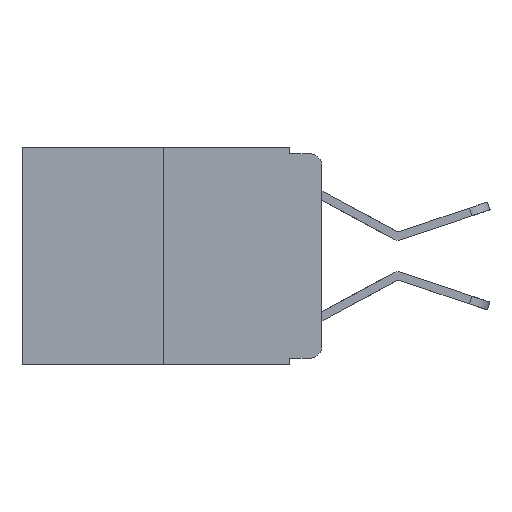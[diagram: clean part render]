
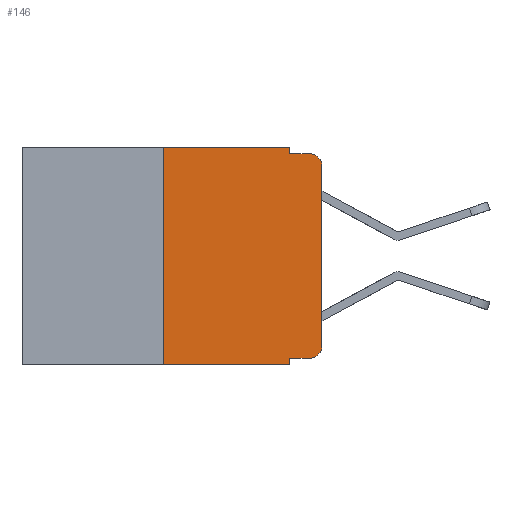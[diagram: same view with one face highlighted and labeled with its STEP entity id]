
A CAD part, left-side view. The second image highlights one B-rep face of the part: STEP entity #146.
In plain terms, the highlighted planar face has unit normal (-1, 0, 0).
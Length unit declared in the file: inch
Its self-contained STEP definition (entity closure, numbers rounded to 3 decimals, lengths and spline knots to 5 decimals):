
#146 = ADVANCED_FACE ( 'NONE', ( #7607 ), #9299, .F. ) ;
#160 = ORIENTED_EDGE ( 'NONE', *, *, #3520, .F. ) ;
#788 = CARTESIAN_POINT ( 'NONE',  ( 0., 0.02, -0.313 ) ) ;
#868 = VECTOR ( 'NONE', #3512, 39.37008 ) ;
#884 = DIRECTION ( 'NONE',  ( 0., 0., -1. ) ) ;
#888 = DIRECTION ( 'NONE',  ( -1., 0., 0. ) ) ;
#1109 = EDGE_CURVE ( 'NONE', #9514, #2259, #11479, .T. ) ;
#1630 = AXIS2_PLACEMENT_3D ( 'NONE', #13753, #9188, #12756 ) ;
#1663 = ORIENTED_EDGE ( 'NONE', *, *, #10226, .F. ) ;
#1716 = EDGE_CURVE ( 'NONE', #8911, #2259, #13193, .T. ) ;
#1800 = CARTESIAN_POINT ( 'NONE',  ( 0., 0.02, -0.01 ) ) ;
#1866 = EDGE_LOOP ( 'NONE', ( #13792, #16588, #160, #4983, #1663, #15312, #2138, #9152, #2629, #4587 ) ) ;
#2138 = ORIENTED_EDGE ( 'NONE', *, *, #1716, .T. ) ;
#2211 = DIRECTION ( 'NONE',  ( 0., 0., -1. ) ) ;
#2259 = VERTEX_POINT ( 'NONE', #12428 ) ;
#2629 = ORIENTED_EDGE ( 'NONE', *, *, #8737, .T. ) ;
#2743 = LINE ( 'NONE', #14825, #12563 ) ;
#2790 = EDGE_CURVE ( 'NONE', #14588, #6689, #4477, .T. ) ;
#3344 = EDGE_CURVE ( 'NONE', #6689, #14003, #9410, .T. ) ;
#3512 = DIRECTION ( 'NONE',  ( 0., -1., 0. ) ) ;
#3520 = EDGE_CURVE ( 'NONE', #7064, #14003, #12764, .T. ) ;
#3581 = EDGE_CURVE ( 'NONE', #12014, #14588, #5286, .T. ) ;
#3714 = EDGE_CURVE ( 'NONE', #14171, #7064, #2743, .T. ) ;
#3899 = EDGE_CURVE ( 'NONE', #8911, #6741, #6055, .T. ) ;
#4477 = LINE ( 'NONE', #5483, #7449 ) ;
#4587 = ORIENTED_EDGE ( 'NONE', *, *, #3581, .T. ) ;
#4983 = ORIENTED_EDGE ( 'NONE', *, *, #3714, .F. ) ;
#5286 = CIRCLE ( 'NONE', #15827, 0.02 ) ;
#5483 = CARTESIAN_POINT ( 'NONE',  ( 0., 0., 0. ) ) ;
#5756 = CARTESIAN_POINT ( 'NONE',  ( 0., 0., -0.313 ) ) ;
#6055 = LINE ( 'NONE', #10056, #12352 ) ;
#6105 = CARTESIAN_POINT ( 'NONE',  ( 0., 0.473, 0. ) ) ;
#6464 = DIRECTION ( 'NONE',  ( 0., -1., 0. ) ) ;
#6689 = VERTEX_POINT ( 'NONE', #10439 ) ;
#6741 = VERTEX_POINT ( 'NONE', #9517 ) ;
#7064 = VERTEX_POINT ( 'NONE', #16178 ) ;
#7449 = VECTOR ( 'NONE', #15978, 39.37008 ) ;
#7607 = FACE_OUTER_BOUND ( 'NONE', #1866, .T. ) ;
#8463 = LINE ( 'NONE', #6105, #868 ) ;
#8737 = EDGE_CURVE ( 'NONE', #9514, #12014, #13579, .T. ) ;
#8911 = VERTEX_POINT ( 'NONE', #13005 ) ;
#9152 = ORIENTED_EDGE ( 'NONE', *, *, #1109, .F. ) ;
#9188 = DIRECTION ( 'NONE',  ( 1., 0., 0. ) ) ;
#9299 = PLANE ( 'NONE',  #1630 ) ;
#9410 = CIRCLE ( 'NONE', #14529, 0.02 ) ;
#9514 = VERTEX_POINT ( 'NONE', #12616 ) ;
#9517 = CARTESIAN_POINT ( 'NONE',  ( 0., 0.25, 0. ) ) ;
#9682 = DIRECTION ( 'NONE',  ( 0., 0., 1. ) ) ;
#9866 = DIRECTION ( 'NONE',  ( 0., 0., -1. ) ) ;
#10056 = CARTESIAN_POINT ( 'NONE',  ( 0., 0.25, 0. ) ) ;
#10219 = CARTESIAN_POINT ( 'NONE',  ( 0., 0.051, -0.333 ) ) ;
#10226 = EDGE_CURVE ( 'NONE', #6741, #14171, #8463, .T. ) ;
#10268 = VECTOR ( 'NONE', #11084, 39.37008 ) ;
#10271 = VECTOR ( 'NONE', #6464, 39.37008 ) ;
#10439 = CARTESIAN_POINT ( 'NONE',  ( 0., 0., -0.03 ) ) ;
#11084 = DIRECTION ( 'NONE',  ( 0., -1., 0. ) ) ;
#11479 = LINE ( 'NONE', #12471, #14338 ) ;
#12014 = VERTEX_POINT ( 'NONE', #14206 ) ;
#12249 = CARTESIAN_POINT ( 'NONE',  ( 0., 0.02, -0.03 ) ) ;
#12352 = VECTOR ( 'NONE', #9682, 39.37008 ) ;
#12369 = VECTOR ( 'NONE', #15624, 39.37008 ) ;
#12428 = CARTESIAN_POINT ( 'NONE',  ( 0., 0.051, -0.343 ) ) ;
#12471 = CARTESIAN_POINT ( 'NONE',  ( 0., 0.051, 0. ) ) ;
#12563 = VECTOR ( 'NONE', #2211, 39.37008 ) ;
#12607 = DIRECTION ( 'NONE',  ( 0., 0., -1. ) ) ;
#12615 = DIRECTION ( 'NONE',  ( -1., 0., 0. ) ) ;
#12616 = CARTESIAN_POINT ( 'NONE',  ( 0., 0.051, -0.333 ) ) ;
#12756 = DIRECTION ( 'NONE',  ( 0., 0., -1. ) ) ;
#12764 = LINE ( 'NONE', #14473, #12369 ) ;
#13005 = CARTESIAN_POINT ( 'NONE',  ( 0., 0.25, -0.343 ) ) ;
#13193 = LINE ( 'NONE', #14553, #10268 ) ;
#13579 = LINE ( 'NONE', #10219, #10271 ) ;
#13753 = CARTESIAN_POINT ( 'NONE',  ( 0., 0.473, 0. ) ) ;
#13792 = ORIENTED_EDGE ( 'NONE', *, *, #2790, .T. ) ;
#14003 = VERTEX_POINT ( 'NONE', #1800 ) ;
#14171 = VERTEX_POINT ( 'NONE', #16099 ) ;
#14206 = CARTESIAN_POINT ( 'NONE',  ( 0., 0.02, -0.333 ) ) ;
#14338 = VECTOR ( 'NONE', #9866, 39.37008 ) ;
#14473 = CARTESIAN_POINT ( 'NONE',  ( 0., 0.051, -0.01 ) ) ;
#14529 = AXIS2_PLACEMENT_3D ( 'NONE', #12249, #12615, #12607 ) ;
#14553 = CARTESIAN_POINT ( 'NONE',  ( 0., 0.473, -0.343 ) ) ;
#14588 = VERTEX_POINT ( 'NONE', #5756 ) ;
#14825 = CARTESIAN_POINT ( 'NONE',  ( 0., 0.051, 0. ) ) ;
#15312 = ORIENTED_EDGE ( 'NONE', *, *, #3899, .F. ) ;
#15624 = DIRECTION ( 'NONE',  ( 0., -1., 0. ) ) ;
#15827 = AXIS2_PLACEMENT_3D ( 'NONE', #788, #888, #884 ) ;
#15978 = DIRECTION ( 'NONE',  ( 0., 0., 1. ) ) ;
#16099 = CARTESIAN_POINT ( 'NONE',  ( 0., 0.051, 0. ) ) ;
#16178 = CARTESIAN_POINT ( 'NONE',  ( 0., 0.051, -0.01 ) ) ;
#16588 = ORIENTED_EDGE ( 'NONE', *, *, #3344, .T. ) ;
